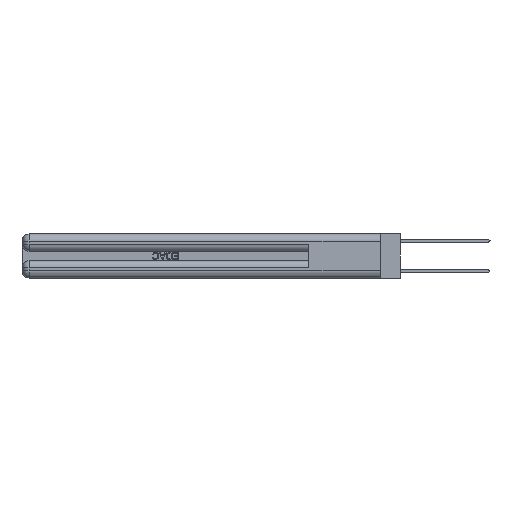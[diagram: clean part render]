
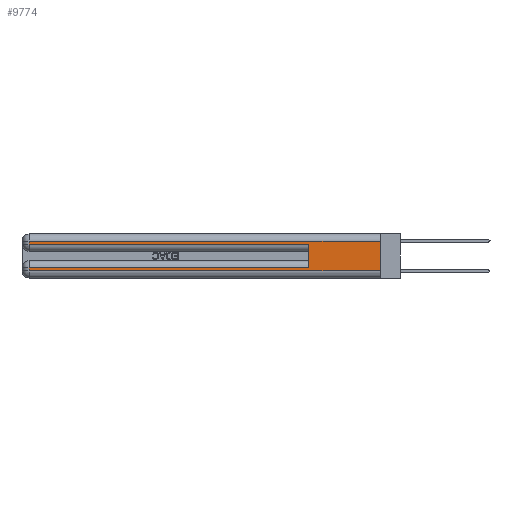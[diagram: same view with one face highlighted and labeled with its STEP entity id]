
A CAD part, left-side view. The second image highlights one B-rep face of the part: STEP entity #9774.
In plain terms, the highlighted planar face has unit normal (-1, 0, 0).
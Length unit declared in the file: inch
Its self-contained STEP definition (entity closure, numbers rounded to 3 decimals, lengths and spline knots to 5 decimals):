
#304 = VERTEX_POINT ( 'NONE', #13323 ) ;
#1247 = ORIENTED_EDGE ( 'NONE', *, *, #5598, .T. ) ;
#1869 = EDGE_CURVE ( 'NONE', #304, #17512, #19825, .T. ) ;
#2422 = CARTESIAN_POINT ( 'NONE',  ( 0., 0., 0.285 ) ) ;
#2569 = CARTESIAN_POINT ( 'NONE',  ( 0., 0., 0.085 ) ) ;
#3969 = ORIENTED_EDGE ( 'NONE', *, *, #32067, .T. ) ;
#5329 = CARTESIAN_POINT ( 'NONE',  ( 0., 0.6, 0.285 ) ) ;
#5598 = EDGE_CURVE ( 'NONE', #25781, #17600, #12165, .T. ) ;
#5706 = CARTESIAN_POINT ( 'NONE',  ( 0., 0.6, 0.145 ) ) ;
#5881 = CARTESIAN_POINT ( 'NONE',  ( 0., 0., 0.31 ) ) ;
#6059 = DIRECTION ( 'NONE',  ( 0., 1., 0. ) ) ;
#7035 = LINE ( 'NONE', #24059, #12163 ) ;
#9184 = DIRECTION ( 'NONE',  ( 0., 0., -1. ) ) ;
#9679 = VECTOR ( 'NONE', #6059, 39.37008 ) ;
#9750 = DIRECTION ( 'NONE',  ( 0., 0., -1. ) ) ;
#9774 = ADVANCED_FACE ( 'NONE', ( #24270 ), #10672, .F. ) ;
#10657 = ORIENTED_EDGE ( 'NONE', *, *, #1869, .T. ) ;
#10672 = PLANE ( 'NONE',  #22367 ) ;
#12163 = VECTOR ( 'NONE', #9750, 39.37008 ) ;
#12165 = LINE ( 'NONE', #25590, #29848 ) ;
#12231 = CARTESIAN_POINT ( 'NONE',  ( 0., 2.94, 0.31 ) ) ;
#12946 = DIRECTION ( 'NONE',  ( 0., -1., 0. ) ) ;
#13323 = CARTESIAN_POINT ( 'NONE',  ( 0., 0., 0.31 ) ) ;
#13946 = VECTOR ( 'NONE', #21238, 39.37008 ) ;
#14031 = DIRECTION ( 'NONE',  ( 0., -1., 0. ) ) ;
#15523 = EDGE_CURVE ( 'NONE', #17512, #16998, #22962, .T. ) ;
#16480 = EDGE_CURVE ( 'NONE', #17600, #21843, #33576, .T. ) ;
#16998 = VERTEX_POINT ( 'NONE', #23506 ) ;
#17512 = VERTEX_POINT ( 'NONE', #12231 ) ;
#17600 = VERTEX_POINT ( 'NONE', #22001 ) ;
#18470 = VECTOR ( 'NONE', #12946, 39.37008 ) ;
#18776 = VECTOR ( 'NONE', #9184, 39.37008 ) ;
#19421 = ORIENTED_EDGE ( 'NONE', *, *, #33727, .T. ) ;
#19825 = LINE ( 'NONE', #5881, #9679 ) ;
#20839 = EDGE_LOOP ( 'NONE', ( #30803, #10657, #29597, #3969, #28570, #19421, #1247, #34813 ) ) ;
#21238 = DIRECTION ( 'NONE',  ( 0., 1., 0. ) ) ;
#21543 = DIRECTION ( 'NONE',  ( 0., 0., -1. ) ) ;
#21620 = VECTOR ( 'NONE', #14031, 39.37008 ) ;
#21843 = VERTEX_POINT ( 'NONE', #32030 ) ;
#22001 = CARTESIAN_POINT ( 'NONE',  ( 0., 2.94, 0.06 ) ) ;
#22356 = CARTESIAN_POINT ( 'NONE',  ( 0., 0., 0.06 ) ) ;
#22367 = AXIS2_PLACEMENT_3D ( 'NONE', #33144, #35326, #21543 ) ;
#22962 = LINE ( 'NONE', #34018, #18776 ) ;
#23146 = EDGE_CURVE ( 'NONE', #304, #21843, #7035, .T. ) ;
#23506 = CARTESIAN_POINT ( 'NONE',  ( 0., 2.94, 0.285 ) ) ;
#24059 = CARTESIAN_POINT ( 'NONE',  ( 0., 0., 0.37 ) ) ;
#24270 = FACE_OUTER_BOUND ( 'NONE', #20839, .T. ) ;
#24351 = LINE ( 'NONE', #2422, #18470 ) ;
#24917 = DIRECTION ( 'NONE',  ( 0., 0., 1. ) ) ;
#25590 = CARTESIAN_POINT ( 'NONE',  ( 0., 2.94, 0.37 ) ) ;
#25781 = VERTEX_POINT ( 'NONE', #29444 ) ;
#25921 = EDGE_CURVE ( 'NONE', #29764, #28467, #30531, .T. ) ;
#28467 = VERTEX_POINT ( 'NONE', #5329 ) ;
#28570 = ORIENTED_EDGE ( 'NONE', *, *, #25921, .F. ) ;
#28844 = DIRECTION ( 'NONE',  ( 0., 0., -1. ) ) ;
#29444 = CARTESIAN_POINT ( 'NONE',  ( 0., 2.94, 0.085 ) ) ;
#29567 = LINE ( 'NONE', #2569, #13946 ) ;
#29597 = ORIENTED_EDGE ( 'NONE', *, *, #15523, .T. ) ;
#29764 = VERTEX_POINT ( 'NONE', #31285 ) ;
#29848 = VECTOR ( 'NONE', #28844, 39.37008 ) ;
#30531 = LINE ( 'NONE', #5706, #35474 ) ;
#30803 = ORIENTED_EDGE ( 'NONE', *, *, #23146, .F. ) ;
#31285 = CARTESIAN_POINT ( 'NONE',  ( 0., 0.6, 0.085 ) ) ;
#32030 = CARTESIAN_POINT ( 'NONE',  ( 0., 0., 0.06 ) ) ;
#32067 = EDGE_CURVE ( 'NONE', #16998, #28467, #24351, .T. ) ;
#33144 = CARTESIAN_POINT ( 'NONE',  ( 0., 0., 0.37 ) ) ;
#33576 = LINE ( 'NONE', #22356, #21620 ) ;
#33727 = EDGE_CURVE ( 'NONE', #29764, #25781, #29567, .T. ) ;
#34018 = CARTESIAN_POINT ( 'NONE',  ( 0., 2.94, 0.37 ) ) ;
#34813 = ORIENTED_EDGE ( 'NONE', *, *, #16480, .T. ) ;
#35326 = DIRECTION ( 'NONE',  ( 1., 0., 0. ) ) ;
#35474 = VECTOR ( 'NONE', #24917, 39.37008 ) ;
